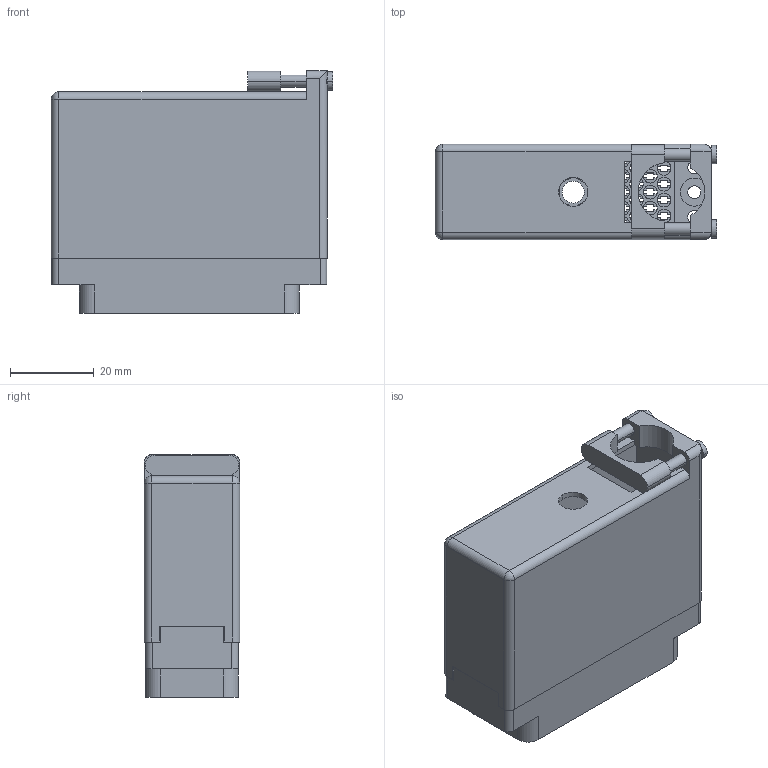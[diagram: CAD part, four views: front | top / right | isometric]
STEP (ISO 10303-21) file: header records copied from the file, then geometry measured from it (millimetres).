
FILE_DESCRIPTION (( 'STEP AP203' ), '1' );
FILE_NAME ('516-056-000-160.STEP', '2020-03-10T04:16:07', ( '' ), ( '' ), 'SwSTEP 2.0', 'SolidWorks 2016', '' );
FILE_SCHEMA (( 'CONFIG_CONTROL_DESIGN' ));
Length unit declared in the file: inch
Products named in the file (3): 516-056-000-160; 516-230-001_Metal - 056 Top Entry; 516 Plug Insulator_056
Assembly tree (2 placements, depth 2):
  516-056-000-160
    516 Plug Insulator_056
    516-230-001_Metal - 056 Top Entry
Bounding box: 67.31 x 22.83 x 58.12 mm (x, y, z)
Volume: 21832.2 mm3; surface area: 31978.3 mm2
Topology: 2 solids, 2 shells, 1281 faces, 3772 edges, 2508 vertices
Faces by surface type: plane 930, cylinder 347, cone 2, sphere 2
Entity records: 43225 total; most frequent: CARTESIAN_POINT 7606, ORIENTED_EDGE 7540, DIRECTION 7254, EDGE_CURVE 3770, VECTOR 2846, LINE 2846, VERTEX_POINT 2508, AXIS2_PLACEMENT_3D 2204
